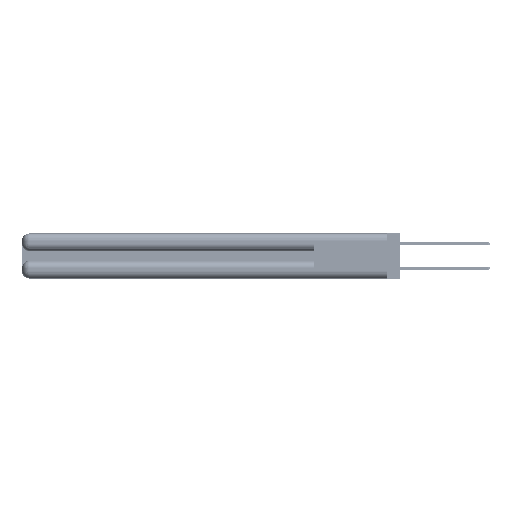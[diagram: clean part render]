
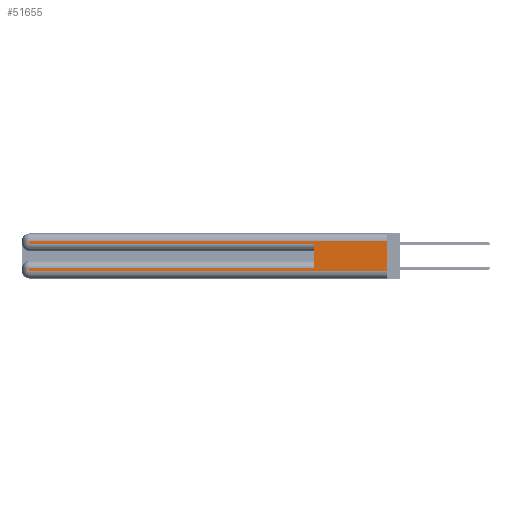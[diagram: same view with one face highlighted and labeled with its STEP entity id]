
A CAD part, left-side view. The second image highlights one B-rep face of the part: STEP entity #51655.
In plain terms, the highlighted planar face has unit normal (-1, 0, 0).
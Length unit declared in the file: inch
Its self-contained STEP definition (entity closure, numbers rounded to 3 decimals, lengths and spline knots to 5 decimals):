
#2222 = EDGE_CURVE ( 'NONE', #3844, #56247, #46151, .T. ) ;
#2922 = VERTEX_POINT ( 'NONE', #17562 ) ;
#3843 = CARTESIAN_POINT ( 'NONE',  ( 0., 2.94, 0.37 ) ) ;
#3844 = VERTEX_POINT ( 'NONE', #4259 ) ;
#4077 = CARTESIAN_POINT ( 'NONE',  ( 0., 0., 0.37 ) ) ;
#4247 = CARTESIAN_POINT ( 'NONE',  ( 0., 0., 0.31 ) ) ;
#4259 = CARTESIAN_POINT ( 'NONE',  ( 0., 0., 0.31 ) ) ;
#6280 = LINE ( 'NONE', #36156, #16552 ) ;
#6608 = ORIENTED_EDGE ( 'NONE', *, *, #2222, .T. ) ;
#6618 = CARTESIAN_POINT ( 'NONE',  ( 0., 0.6, 0.085 ) ) ;
#6833 = ORIENTED_EDGE ( 'NONE', *, *, #22619, .T. ) ;
#7910 = VERTEX_POINT ( 'NONE', #6618 ) ;
#8263 = DIRECTION ( 'NONE',  ( 0., -1., 0. ) ) ;
#9491 = CARTESIAN_POINT ( 'NONE',  ( 0., 2.94, 0.31 ) ) ;
#9859 = LINE ( 'NONE', #52571, #44037 ) ;
#10056 = LINE ( 'NONE', #16736, #36687 ) ;
#11336 = VECTOR ( 'NONE', #34920, 39.37008 ) ;
#11834 = ORIENTED_EDGE ( 'NONE', *, *, #36337, .F. ) ;
#12507 = EDGE_CURVE ( 'NONE', #13777, #44209, #10056, .T. ) ;
#12933 = CARTESIAN_POINT ( 'NONE',  ( 0., 0.6, 0.285 ) ) ;
#13249 = EDGE_CURVE ( 'NONE', #56247, #13777, #48852, .T. ) ;
#13777 = VERTEX_POINT ( 'NONE', #34563 ) ;
#16552 = VECTOR ( 'NONE', #40560, 39.37008 ) ;
#16736 = CARTESIAN_POINT ( 'NONE',  ( 0., 0., 0.285 ) ) ;
#16790 = VECTOR ( 'NONE', #43137, 39.37008 ) ;
#17269 = DIRECTION ( 'NONE',  ( 0., -1., 0. ) ) ;
#17562 = CARTESIAN_POINT ( 'NONE',  ( 0., 2.94, 0.085 ) ) ;
#19678 = LINE ( 'NONE', #51141, #48986 ) ;
#20283 = EDGE_CURVE ( 'NONE', #2922, #54168, #6280, .T. ) ;
#21045 = ORIENTED_EDGE ( 'NONE', *, *, #13249, .T. ) ;
#21329 = CARTESIAN_POINT ( 'NONE',  ( 0., 0., 0.085 ) ) ;
#22207 = ORIENTED_EDGE ( 'NONE', *, *, #45373, .T. ) ;
#22619 = EDGE_CURVE ( 'NONE', #54168, #45158, #39649, .T. ) ;
#24019 = CARTESIAN_POINT ( 'NONE',  ( 0., 0., 0.06 ) ) ;
#24168 = EDGE_LOOP ( 'NONE', ( #11834, #6608, #21045, #46604, #48593, #22207, #33479, #6833 ) ) ;
#24660 = EDGE_CURVE ( 'NONE', #7910, #44209, #19678, .T. ) ;
#25453 = VECTOR ( 'NONE', #34255, 39.37008 ) ;
#30906 = LINE ( 'NONE', #21329, #25453 ) ;
#32787 = VECTOR ( 'NONE', #17269, 39.37008 ) ;
#33479 = ORIENTED_EDGE ( 'NONE', *, *, #20283, .T. ) ;
#34187 = DIRECTION ( 'NONE',  ( 1., 0., 0. ) ) ;
#34255 = DIRECTION ( 'NONE',  ( 0., 1., 0. ) ) ;
#34563 = CARTESIAN_POINT ( 'NONE',  ( 0., 2.94, 0.285 ) ) ;
#34920 = DIRECTION ( 'NONE',  ( 0., 1., 0. ) ) ;
#36156 = CARTESIAN_POINT ( 'NONE',  ( 0., 2.94, 0.37 ) ) ;
#36337 = EDGE_CURVE ( 'NONE', #3844, #45158, #9859, .T. ) ;
#36687 = VECTOR ( 'NONE', #8263, 39.37008 ) ;
#38393 = FACE_OUTER_BOUND ( 'NONE', #24168, .T. ) ;
#38789 = PLANE ( 'NONE',  #46908 ) ;
#39649 = LINE ( 'NONE', #47759, #32787 ) ;
#40560 = DIRECTION ( 'NONE',  ( 0., 0., -1. ) ) ;
#43137 = DIRECTION ( 'NONE',  ( 0., 0., -1. ) ) ;
#43373 = DIRECTION ( 'NONE',  ( 0., 0., -1. ) ) ;
#44037 = VECTOR ( 'NONE', #54083, 39.37008 ) ;
#44209 = VERTEX_POINT ( 'NONE', #12933 ) ;
#45158 = VERTEX_POINT ( 'NONE', #24019 ) ;
#45373 = EDGE_CURVE ( 'NONE', #7910, #2922, #30906, .T. ) ;
#46151 = LINE ( 'NONE', #4247, #11336 ) ;
#46178 = CARTESIAN_POINT ( 'NONE',  ( 0., 2.94, 0.06 ) ) ;
#46604 = ORIENTED_EDGE ( 'NONE', *, *, #12507, .T. ) ;
#46908 = AXIS2_PLACEMENT_3D ( 'NONE', #4077, #34187, #43373 ) ;
#47759 = CARTESIAN_POINT ( 'NONE',  ( 0., 0., 0.06 ) ) ;
#48593 = ORIENTED_EDGE ( 'NONE', *, *, #24660, .F. ) ;
#48852 = LINE ( 'NONE', #3843, #16790 ) ;
#48986 = VECTOR ( 'NONE', #55501, 39.37008 ) ;
#51141 = CARTESIAN_POINT ( 'NONE',  ( 0., 0.6, 0.145 ) ) ;
#51655 = ADVANCED_FACE ( 'NONE', ( #38393 ), #38789, .F. ) ;
#52571 = CARTESIAN_POINT ( 'NONE',  ( 0., 0., 0.37 ) ) ;
#54083 = DIRECTION ( 'NONE',  ( 0., 0., -1. ) ) ;
#54168 = VERTEX_POINT ( 'NONE', #46178 ) ;
#55501 = DIRECTION ( 'NONE',  ( 0., 0., 1. ) ) ;
#56247 = VERTEX_POINT ( 'NONE', #9491 ) ;
